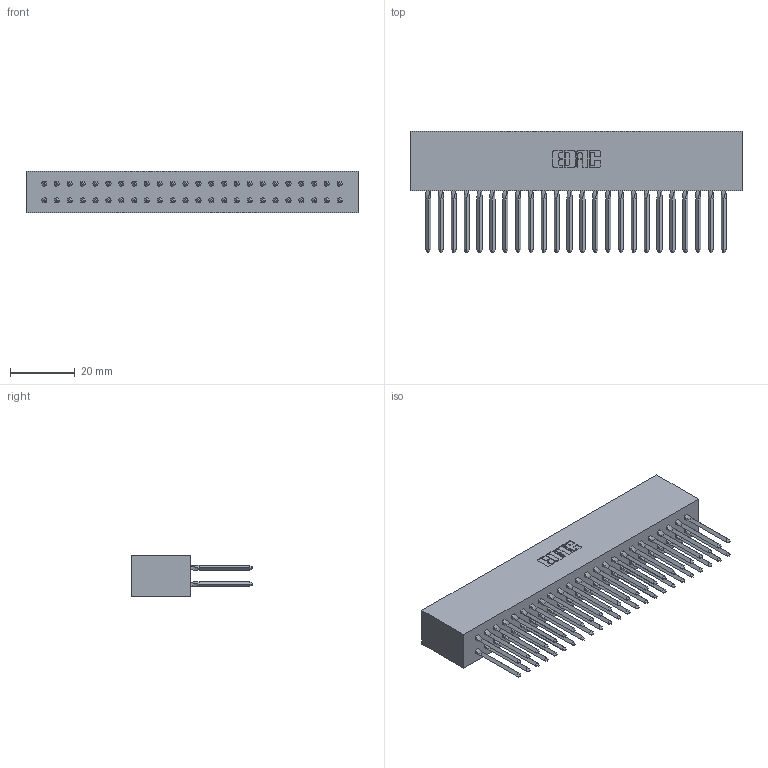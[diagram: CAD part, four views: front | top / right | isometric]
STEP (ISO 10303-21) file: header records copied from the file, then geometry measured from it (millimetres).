
FILE_DESCRIPTION (( 'STEP AP203' ), '1' );
FILE_NAME ('317-048-542-801.STEP', '2020-02-28T02:46:53', ( '' ), ( '' ), 'SwSTEP 2.0', 'SolidWorks 2016', '' );
FILE_SCHEMA (( 'CONFIG_CONTROL_DESIGN' ));
Length unit declared in the file: inch
Products named in the file (3): 317 Part_Lugless; 317-048-542-801; 317-290-003_542
Assembly tree (49 placements, depth 2):
  317-048-542-801
    317 Part_Lugless
    317-290-003_542  x48
Bounding box: 102.31 x 37.34 x 12.7 mm (x, y, z)
Volume: 17914.6 mm3; surface area: 24511 mm2
Topology: 49 solids, 49 shells, 2826 faces, 7919 edges, 5054 vertices
Faces by surface type: plane 2258, cylinder 376, bspline 192
Entity records: 35811 total; most frequent: CARTESIAN_POINT 6493, ORIENTED_EDGE 6156, DIRECTION 5202, EDGE_CURVE 3078, LINE 2916, VECTOR 2916, VERTEX_POINT 2046, AXIS2_PLACEMENT_3D 1143
